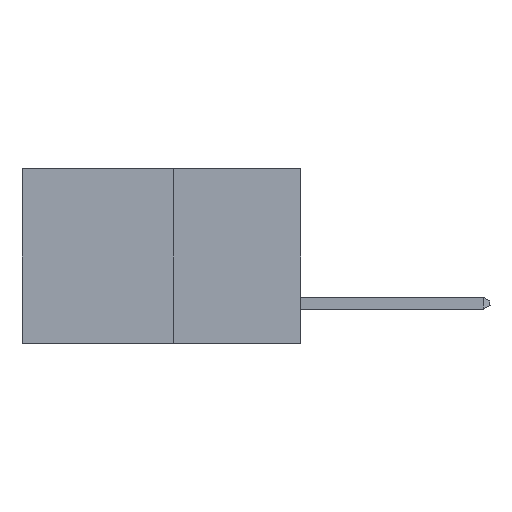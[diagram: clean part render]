
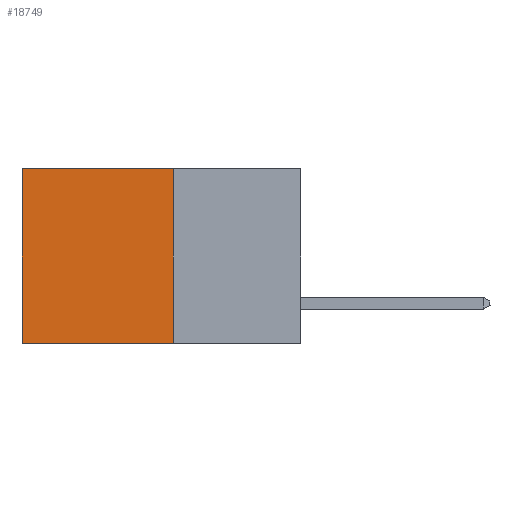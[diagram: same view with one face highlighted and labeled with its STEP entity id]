
A CAD part, left-side view. The second image highlights one B-rep face of the part: STEP entity #18749.
In plain terms, the highlighted planar face has unit normal (-1, 0, 0).
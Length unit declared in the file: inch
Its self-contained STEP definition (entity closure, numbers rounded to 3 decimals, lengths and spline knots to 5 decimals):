
#150 = DIRECTION ( 'NONE',  ( 0., 0., -1. ) ) ;
#657 = PLANE ( 'NONE',  #13844 ) ;
#1204 = VERTEX_POINT ( 'NONE', #2590 ) ;
#2208 = EDGE_CURVE ( 'NONE', #6490, #1204, #7823, .T. ) ;
#2590 = CARTESIAN_POINT ( 'NONE',  ( 0.277, 0.59, -0.37 ) ) ;
#2625 = ORIENTED_EDGE ( 'NONE', *, *, #13446, .F. ) ;
#3187 = CARTESIAN_POINT ( 'NONE',  ( 0.277, 0.27, 0. ) ) ;
#3241 = DIRECTION ( 'NONE',  ( 0., 1., 0. ) ) ;
#3976 = CARTESIAN_POINT ( 'NONE',  ( 0.277, 0.27, 0. ) ) ;
#4041 = LINE ( 'NONE', #15471, #15311 ) ;
#4356 = VECTOR ( 'NONE', #15810, 39.37008 ) ;
#4965 = VERTEX_POINT ( 'NONE', #3187 ) ;
#5026 = DIRECTION ( 'NONE',  ( 1., 0., 0. ) ) ;
#5041 = EDGE_LOOP ( 'NONE', ( #14728, #16882, #2625, #16131 ) ) ;
#5197 = EDGE_CURVE ( 'NONE', #4965, #6490, #13520, .T. ) ;
#5205 = VECTOR ( 'NONE', #3241, 39.37008 ) ;
#5603 = FACE_OUTER_BOUND ( 'NONE', #5041, .T. ) ;
#6490 = VERTEX_POINT ( 'NONE', #13762 ) ;
#7526 = VECTOR ( 'NONE', #150, 39.37008 ) ;
#7823 = LINE ( 'NONE', #14264, #4356 ) ;
#8937 = CARTESIAN_POINT ( 'NONE',  ( 0.277, 0.27, -0.37 ) ) ;
#13446 = EDGE_CURVE ( 'NONE', #4965, #17582, #15364, .T. ) ;
#13520 = LINE ( 'NONE', #3976, #5205 ) ;
#13762 = CARTESIAN_POINT ( 'NONE',  ( 0.277, 0.59, 0. ) ) ;
#13844 = AXIS2_PLACEMENT_3D ( 'NONE', #13865, #5026, #15308 ) ;
#13865 = CARTESIAN_POINT ( 'NONE',  ( 0.277, 0.27, -0.37 ) ) ;
#14264 = CARTESIAN_POINT ( 'NONE',  ( 0.277, 0.59, -0.37 ) ) ;
#14728 = ORIENTED_EDGE ( 'NONE', *, *, #2208, .T. ) ;
#15308 = DIRECTION ( 'NONE',  ( 0., 0., -1. ) ) ;
#15311 = VECTOR ( 'NONE', #18378, 39.37008 ) ;
#15346 = EDGE_CURVE ( 'NONE', #17582, #1204, #4041, .T. ) ;
#15364 = LINE ( 'NONE', #8937, #7526 ) ;
#15471 = CARTESIAN_POINT ( 'NONE',  ( 0.277, 0.27, -0.37 ) ) ;
#15810 = DIRECTION ( 'NONE',  ( 0., 0., -1. ) ) ;
#16131 = ORIENTED_EDGE ( 'NONE', *, *, #5197, .T. ) ;
#16206 = CARTESIAN_POINT ( 'NONE',  ( 0.277, 0.27, -0.37 ) ) ;
#16882 = ORIENTED_EDGE ( 'NONE', *, *, #15346, .F. ) ;
#17582 = VERTEX_POINT ( 'NONE', #16206 ) ;
#18378 = DIRECTION ( 'NONE',  ( 0., 1., 0. ) ) ;
#18749 = ADVANCED_FACE ( 'NONE', ( #5603 ), #657, .F. ) ;
